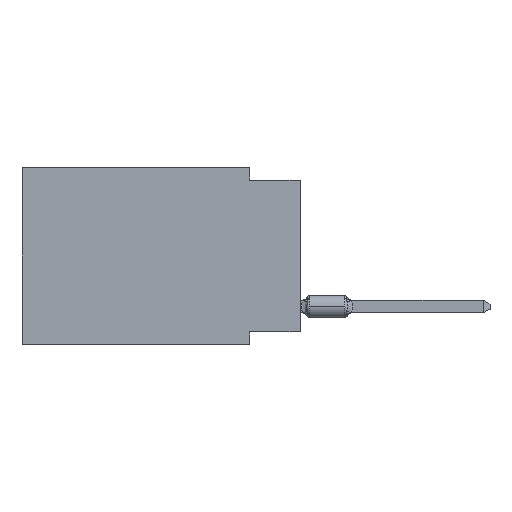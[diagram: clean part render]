
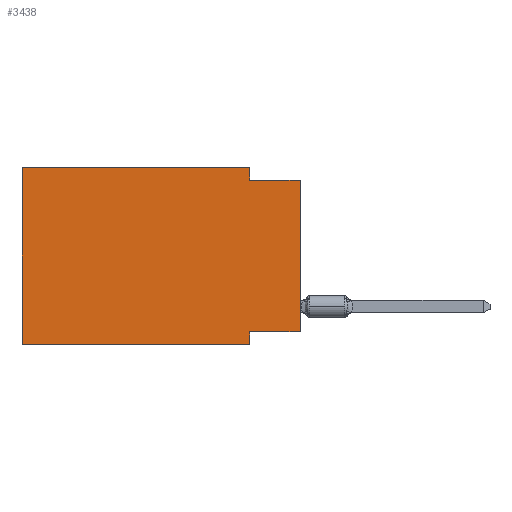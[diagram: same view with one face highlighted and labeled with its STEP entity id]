
A CAD part, left-side view. The second image highlights one B-rep face of the part: STEP entity #3438.
In plain terms, the highlighted planar face has unit normal (-1, 0, 0).
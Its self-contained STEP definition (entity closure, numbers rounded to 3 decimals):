
#43 = CARTESIAN_POINT ( 'NONE',  ( 0., 0., -0.635 ) ) ;
#496 = VECTOR ( 'NONE', #7429, 1000. ) ;
#601 = EDGE_CURVE ( 'NONE', #11739, #1405, #9685, .T. ) ;
#685 = LINE ( 'NONE', #10805, #496 ) ;
#906 = PLANE ( 'NONE',  #12575 ) ;
#1101 = DIRECTION ( 'NONE',  ( 0., 0., 1. ) ) ;
#1405 = VERTEX_POINT ( 'NONE', #3967 ) ;
#1845 = ORIENTED_EDGE ( 'NONE', *, *, #11456, .T. ) ;
#2087 = EDGE_CURVE ( 'NONE', #12540, #7143, #685, .T. ) ;
#2562 = CARTESIAN_POINT ( 'NONE',  ( 0., 2.54, -0.635 ) ) ;
#2690 = DIRECTION ( 'NONE',  ( 0., -1., 0. ) ) ;
#3065 = VECTOR ( 'NONE', #2690, 1000. ) ;
#3105 = VERTEX_POINT ( 'NONE', #43 ) ;
#3208 = VERTEX_POINT ( 'NONE', #2562 ) ;
#3209 = VERTEX_POINT ( 'NONE', #13886 ) ;
#3322 = DIRECTION ( 'NONE',  ( 0., -1., 0. ) ) ;
#3345 = VECTOR ( 'NONE', #8129, 1000. ) ;
#3438 = ADVANCED_FACE ( 'NONE', ( #14626 ), #906, .F. ) ;
#3737 = VECTOR ( 'NONE', #12867, 1000. ) ;
#3808 = VECTOR ( 'NONE', #1101, 1000. ) ;
#3823 = CARTESIAN_POINT ( 'NONE',  ( 0., 2.54, -8.255 ) ) ;
#3967 = CARTESIAN_POINT ( 'NONE',  ( 0., 2.54, -8.89 ) ) ;
#4515 = DIRECTION ( 'NONE',  ( 1., 0., 0. ) ) ;
#4692 = LINE ( 'NONE', #5882, #3345 ) ;
#5550 = LINE ( 'NONE', #10109, #12841 ) ;
#5814 = EDGE_CURVE ( 'NONE', #3208, #3105, #6060, .T. ) ;
#5882 = CARTESIAN_POINT ( 'NONE',  ( 0., 2.54, -8.89 ) ) ;
#6003 = ORIENTED_EDGE ( 'NONE', *, *, #601, .T. ) ;
#6060 = LINE ( 'NONE', #10691, #3065 ) ;
#6081 = EDGE_CURVE ( 'NONE', #11739, #12511, #10162, .T. ) ;
#6570 = CARTESIAN_POINT ( 'NONE',  ( 0., 13.97, -8.89 ) ) ;
#6666 = EDGE_CURVE ( 'NONE', #7143, #1405, #4692, .T. ) ;
#6797 = CARTESIAN_POINT ( 'NONE',  ( 0., 13.97, 0. ) ) ;
#6904 = VECTOR ( 'NONE', #3322, 1000. ) ;
#6921 = EDGE_LOOP ( 'NONE', ( #1845, #8341, #8820, #9115, #12107, #6003, #9605, #10965 ) ) ;
#7143 = VERTEX_POINT ( 'NONE', #3823 ) ;
#7429 = DIRECTION ( 'NONE',  ( 0., 1., 0. ) ) ;
#7466 = CARTESIAN_POINT ( 'NONE',  ( 0., 2.54, 0. ) ) ;
#8032 = EDGE_CURVE ( 'NONE', #12511, #3209, #12372, .T. ) ;
#8129 = DIRECTION ( 'NONE',  ( 0., 0., -1. ) ) ;
#8341 = ORIENTED_EDGE ( 'NONE', *, *, #5814, .F. ) ;
#8564 = DIRECTION ( 'NONE',  ( 0., -1., 0. ) ) ;
#8585 = CARTESIAN_POINT ( 'NONE',  ( 0., 13.97, 0. ) ) ;
#8820 = ORIENTED_EDGE ( 'NONE', *, *, #10466, .F. ) ;
#9115 = ORIENTED_EDGE ( 'NONE', *, *, #8032, .F. ) ;
#9605 = ORIENTED_EDGE ( 'NONE', *, *, #6666, .F. ) ;
#9685 = LINE ( 'NONE', #12014, #12230 ) ;
#10109 = CARTESIAN_POINT ( 'NONE',  ( 0., 0., 0. ) ) ;
#10162 = LINE ( 'NONE', #6797, #3808 ) ;
#10270 = CARTESIAN_POINT ( 'NONE',  ( 0., 13.97, 0. ) ) ;
#10466 = EDGE_CURVE ( 'NONE', #3209, #3208, #13176, .T. ) ;
#10691 = CARTESIAN_POINT ( 'NONE',  ( 0., 0., -0.635 ) ) ;
#10805 = CARTESIAN_POINT ( 'NONE',  ( 0., 0., -8.255 ) ) ;
#10965 = ORIENTED_EDGE ( 'NONE', *, *, #2087, .F. ) ;
#11125 = CARTESIAN_POINT ( 'NONE',  ( 0., 0., -8.255 ) ) ;
#11456 = EDGE_CURVE ( 'NONE', #12540, #3105, #5550, .T. ) ;
#11739 = VERTEX_POINT ( 'NONE', #6570 ) ;
#12014 = CARTESIAN_POINT ( 'NONE',  ( 0., 13.97, -8.89 ) ) ;
#12107 = ORIENTED_EDGE ( 'NONE', *, *, #6081, .F. ) ;
#12230 = VECTOR ( 'NONE', #8564, 1000. ) ;
#12372 = LINE ( 'NONE', #13652, #6904 ) ;
#12511 = VERTEX_POINT ( 'NONE', #8585 ) ;
#12540 = VERTEX_POINT ( 'NONE', #11125 ) ;
#12575 = AXIS2_PLACEMENT_3D ( 'NONE', #10270, #4515, #12586 ) ;
#12586 = DIRECTION ( 'NONE',  ( 0., 0., -1. ) ) ;
#12841 = VECTOR ( 'NONE', #14683, 1000. ) ;
#12867 = DIRECTION ( 'NONE',  ( 0., 0., -1. ) ) ;
#13176 = LINE ( 'NONE', #7466, #3737 ) ;
#13652 = CARTESIAN_POINT ( 'NONE',  ( 0., 13.97, 0. ) ) ;
#13886 = CARTESIAN_POINT ( 'NONE',  ( 0., 2.54, 0. ) ) ;
#14626 = FACE_OUTER_BOUND ( 'NONE', #6921, .T. ) ;
#14683 = DIRECTION ( 'NONE',  ( 0., 0., 1. ) ) ;
